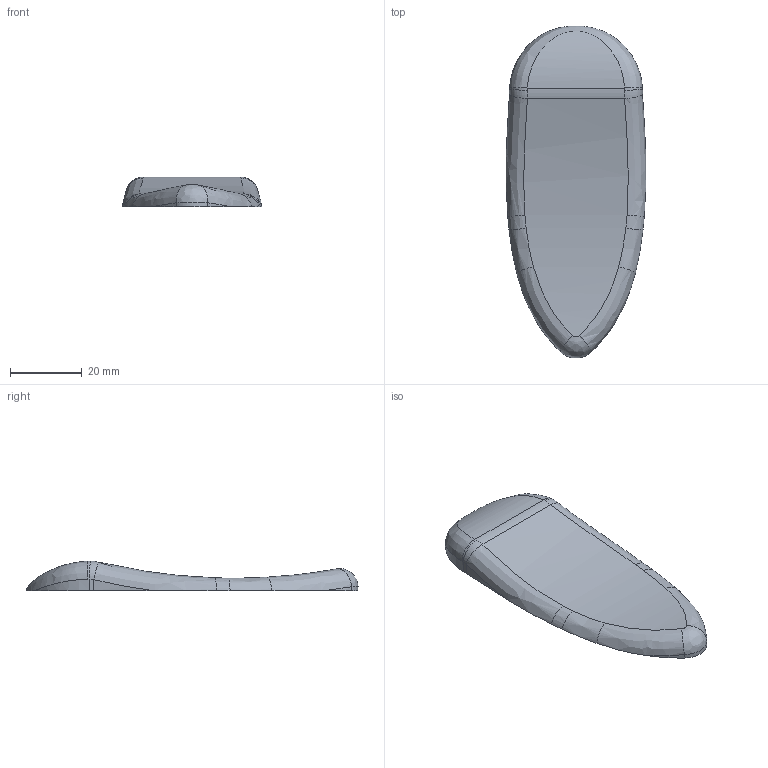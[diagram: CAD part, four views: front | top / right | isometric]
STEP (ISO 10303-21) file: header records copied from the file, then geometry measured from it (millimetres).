
FILE_DESCRIPTION (( 'STEP AP214' ), '1' );
FILE_NAME ('9.STEP', '2013-09-29T07:07:18', ( 'elpi' ), ( '' ), 'SwSTEP 2.0', 'SolidWorks 2013', '' );
FILE_SCHEMA (( 'AUTOMOTIVE_DESIGN' ));
Length unit declared in the file: millimetre
Products named in the file (1): 9
Bounding box: 39.01 x 92.66 x 8.31 mm (x, y, z)
Volume: 14488.3 mm3; surface area: 6680.3 mm2
Topology: 1 solids, 1 shells, 29 faces, 77 edges, 50 vertices
Faces by surface type: bspline 18, torus 4, cylinder 4, plane 3
Entity records: 1643 total; most frequent: CARTESIAN_POINT 1020, ORIENTED_EDGE 154, DIRECTION 78, EDGE_CURVE 77, VERTEX_POINT 50, B_SPLINE_CURVE_WITH_KNOTS 44, AXIS2_PLACEMENT_3D 33, ADVANCED_FACE 29
